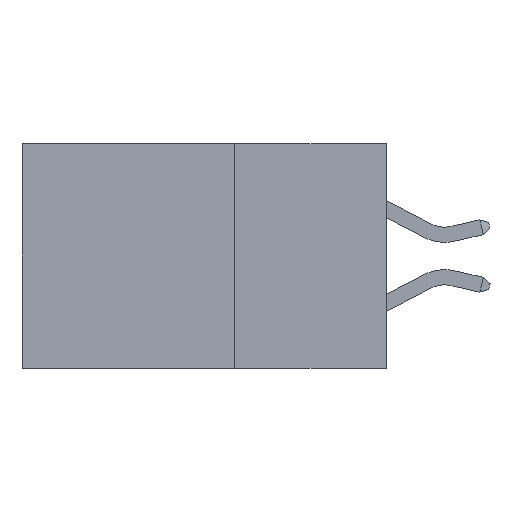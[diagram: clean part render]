
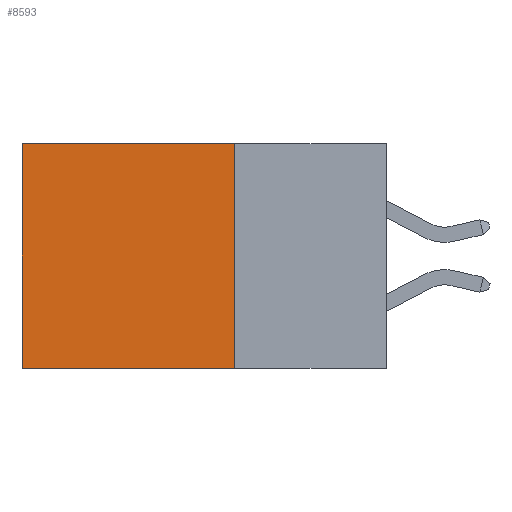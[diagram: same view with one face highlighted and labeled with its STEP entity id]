
A CAD part, left-side view. The second image highlights one B-rep face of the part: STEP entity #8593.
In plain terms, the highlighted planar face has unit normal (-1, 0, 0).
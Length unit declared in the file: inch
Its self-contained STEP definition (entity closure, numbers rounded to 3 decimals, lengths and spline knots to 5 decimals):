
#221 = CARTESIAN_POINT ( 'NONE',  ( 0.298, 0.25, 0. ) ) ;
#925 = CARTESIAN_POINT ( 'NONE',  ( 0.298, 0.25, 0. ) ) ;
#1091 = DIRECTION ( 'NONE',  ( 0., 0., -1. ) ) ;
#1418 = CARTESIAN_POINT ( 'NONE',  ( 0.298, 0.25, 0. ) ) ;
#1797 = FACE_OUTER_BOUND ( 'NONE', #3792, .T. ) ;
#1872 = VECTOR ( 'NONE', #1091, 39.37008 ) ;
#2996 = CARTESIAN_POINT ( 'NONE',  ( 0.298, 0.6, 0. ) ) ;
#3729 = CARTESIAN_POINT ( 'NONE',  ( 0.298, 0.25, 0. ) ) ;
#3746 = CARTESIAN_POINT ( 'NONE',  ( 0.298, 0.6, -0.37 ) ) ;
#3792 = EDGE_LOOP ( 'NONE', ( #9275, #6571, #4151, #8965 ) ) ;
#4034 = DIRECTION ( 'NONE',  ( 0., 1., 0. ) ) ;
#4151 = ORIENTED_EDGE ( 'NONE', *, *, #5243, .F. ) ;
#4728 = VECTOR ( 'NONE', #6528, 39.37008 ) ;
#5135 = LINE ( 'NONE', #221, #4728 ) ;
#5171 = EDGE_CURVE ( 'NONE', #8102, #6346, #8398, .T. ) ;
#5243 = EDGE_CURVE ( 'NONE', #7084, #8240, #9506, .T. ) ;
#5245 = LINE ( 'NONE', #9109, #5972 ) ;
#5788 = EDGE_CURVE ( 'NONE', #7084, #8102, #5135, .T. ) ;
#5972 = VECTOR ( 'NONE', #4034, 39.37008 ) ;
#6346 = VERTEX_POINT ( 'NONE', #3746 ) ;
#6528 = DIRECTION ( 'NONE',  ( 0., 1., 0. ) ) ;
#6571 = ORIENTED_EDGE ( 'NONE', *, *, #7237, .F. ) ;
#7084 = VERTEX_POINT ( 'NONE', #1418 ) ;
#7237 = EDGE_CURVE ( 'NONE', #8240, #6346, #5245, .T. ) ;
#7315 = DIRECTION ( 'NONE',  ( 0., 0., -1. ) ) ;
#8027 = CARTESIAN_POINT ( 'NONE',  ( 0.298, 0.6, 0. ) ) ;
#8095 = VECTOR ( 'NONE', #9711, 39.37008 ) ;
#8102 = VERTEX_POINT ( 'NONE', #2996 ) ;
#8240 = VERTEX_POINT ( 'NONE', #9104 ) ;
#8398 = LINE ( 'NONE', #8027, #8095 ) ;
#8593 = ADVANCED_FACE ( 'NONE', ( #1797 ), #9705, .F. ) ;
#8965 = ORIENTED_EDGE ( 'NONE', *, *, #5788, .T. ) ;
#9024 = DIRECTION ( 'NONE',  ( 1., 0., 0. ) ) ;
#9060 = AXIS2_PLACEMENT_3D ( 'NONE', #925, #9024, #7315 ) ;
#9104 = CARTESIAN_POINT ( 'NONE',  ( 0.298, 0.25, -0.37 ) ) ;
#9109 = CARTESIAN_POINT ( 'NONE',  ( 0.298, 0.25, -0.37 ) ) ;
#9275 = ORIENTED_EDGE ( 'NONE', *, *, #5171, .T. ) ;
#9506 = LINE ( 'NONE', #3729, #1872 ) ;
#9705 = PLANE ( 'NONE',  #9060 ) ;
#9711 = DIRECTION ( 'NONE',  ( 0., 0., -1. ) ) ;
